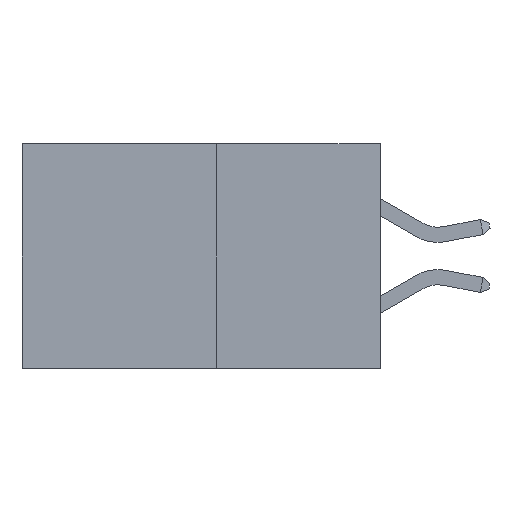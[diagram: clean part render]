
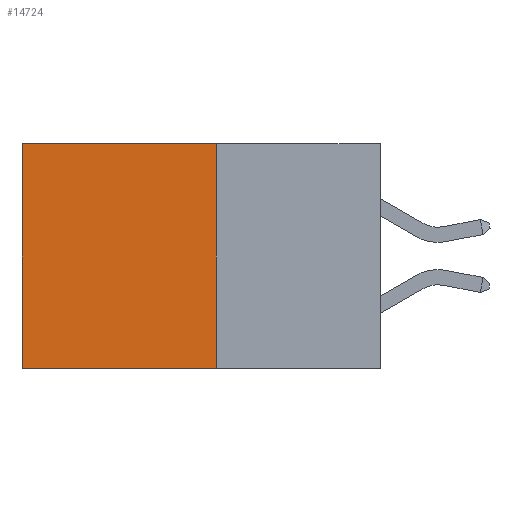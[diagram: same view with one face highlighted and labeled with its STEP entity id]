
A CAD part, left-side view. The second image highlights one B-rep face of the part: STEP entity #14724.
In plain terms, the highlighted planar face has unit normal (-1, 0, 0).
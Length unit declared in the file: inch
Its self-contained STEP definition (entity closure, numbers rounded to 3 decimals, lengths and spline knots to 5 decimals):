
#218 = VERTEX_POINT ( 'NONE', #8920 ) ;
#1540 = VECTOR ( 'NONE', #14427, 39.37008 ) ;
#1827 = AXIS2_PLACEMENT_3D ( 'NONE', #14741, #10683, #6709 ) ;
#3035 = VERTEX_POINT ( 'NONE', #18418 ) ;
#3415 = ORIENTED_EDGE ( 'NONE', *, *, #9702, .F. ) ;
#3747 = VERTEX_POINT ( 'NONE', #12907 ) ;
#5699 = CARTESIAN_POINT ( 'NONE',  ( 0.277, 0.27, 0. ) ) ;
#5881 = LINE ( 'NONE', #16310, #9629 ) ;
#6709 = DIRECTION ( 'NONE',  ( 0., 0., -1. ) ) ;
#6937 = VECTOR ( 'NONE', #13798, 39.37008 ) ;
#7750 = EDGE_CURVE ( 'NONE', #3747, #15689, #5881, .T. ) ;
#8470 = ORIENTED_EDGE ( 'NONE', *, *, #7750, .T. ) ;
#8632 = DIRECTION ( 'NONE',  ( 0., 1., 0. ) ) ;
#8920 = CARTESIAN_POINT ( 'NONE',  ( 0.277, 0.27, 0. ) ) ;
#9089 = PLANE ( 'NONE',  #1827 ) ;
#9629 = VECTOR ( 'NONE', #17706, 39.37008 ) ;
#9702 = EDGE_CURVE ( 'NONE', #3035, #15689, #18106, .T. ) ;
#10247 = ORIENTED_EDGE ( 'NONE', *, *, #10595, .T. ) ;
#10595 = EDGE_CURVE ( 'NONE', #218, #3747, #13916, .T. ) ;
#10683 = DIRECTION ( 'NONE',  ( 1., 0., 0. ) ) ;
#10717 = ORIENTED_EDGE ( 'NONE', *, *, #17983, .F. ) ;
#11810 = FACE_OUTER_BOUND ( 'NONE', #17700, .T. ) ;
#12376 = CARTESIAN_POINT ( 'NONE',  ( 0.277, 0.27, -0.37 ) ) ;
#12907 = CARTESIAN_POINT ( 'NONE',  ( 0.277, 0.59, 0. ) ) ;
#13006 = CARTESIAN_POINT ( 'NONE',  ( 0.277, 0.27, -0.37 ) ) ;
#13032 = LINE ( 'NONE', #13006, #1540 ) ;
#13191 = CARTESIAN_POINT ( 'NONE',  ( 0.277, 0.59, -0.37 ) ) ;
#13798 = DIRECTION ( 'NONE',  ( 0., 1., 0. ) ) ;
#13916 = LINE ( 'NONE', #5699, #17207 ) ;
#14427 = DIRECTION ( 'NONE',  ( 0., 0., -1. ) ) ;
#14724 = ADVANCED_FACE ( 'NONE', ( #11810 ), #9089, .F. ) ;
#14741 = CARTESIAN_POINT ( 'NONE',  ( 0.277, 0.27, -0.37 ) ) ;
#15689 = VERTEX_POINT ( 'NONE', #13191 ) ;
#16310 = CARTESIAN_POINT ( 'NONE',  ( 0.277, 0.59, -0.37 ) ) ;
#17207 = VECTOR ( 'NONE', #8632, 39.37008 ) ;
#17700 = EDGE_LOOP ( 'NONE', ( #8470, #3415, #10717, #10247 ) ) ;
#17706 = DIRECTION ( 'NONE',  ( 0., 0., -1. ) ) ;
#17983 = EDGE_CURVE ( 'NONE', #218, #3035, #13032, .T. ) ;
#18106 = LINE ( 'NONE', #12376, #6937 ) ;
#18418 = CARTESIAN_POINT ( 'NONE',  ( 0.277, 0.27, -0.37 ) ) ;
